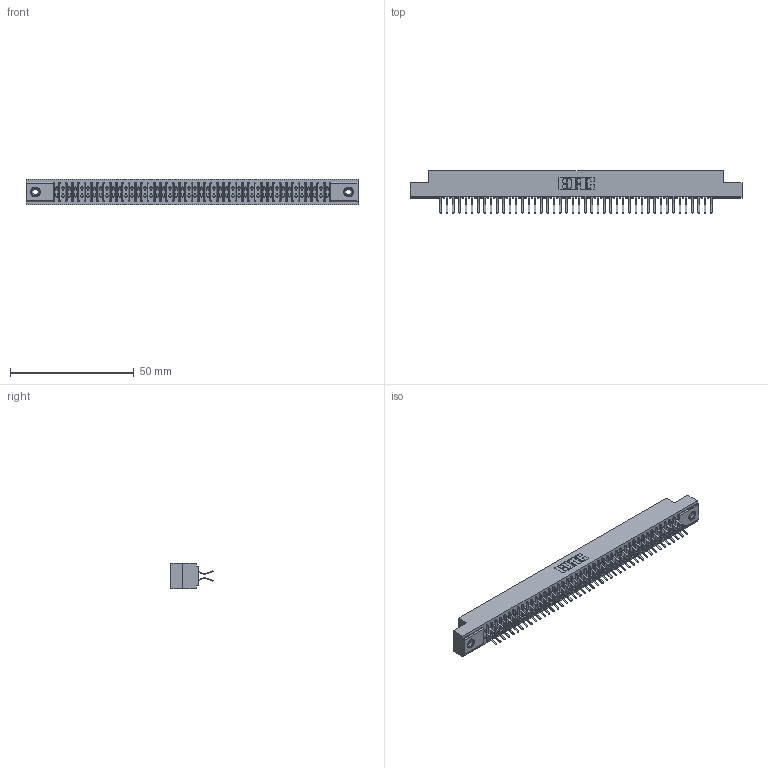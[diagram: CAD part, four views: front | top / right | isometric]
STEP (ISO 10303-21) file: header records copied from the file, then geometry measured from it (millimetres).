
FILE_DESCRIPTION (( 'STEP AP203' ), '1' );
FILE_NAME ('341-088-556-208.STEP', '2018-08-07T23:48:28', ( '' ), ( '' ), 'SwSTEP 2.0', 'SolidWorks 2016', '' );
FILE_SCHEMA (( 'CONFIG_CONTROL_DESIGN' ));
Length unit declared in the file: inch
Products named in the file (4): 341 Part_.156 (3.96) Dia Mounting Holes; 341-292-001_341-292-156; 345-250-001_345-250-003-102; 341-088-556-208
Assembly tree (91 placements, depth 2):
  341-088-556-208
    341 Part_.156 (3.96) Dia Mounting Holes
    341-292-001_341-292-156  x88
    345-250-001_345-250-003-102  x2
Bounding box: 133.99 x 17.07 x 10.16 mm (x, y, z)
Volume: 9917.4 mm3; surface area: 17896.9 mm2
Topology: 91 solids, 91 shells, 6336 faces, 18360 edges, 11906 vertices
Faces by surface type: plane 3620, cylinder 2524, sphere 90, torus 90, cone 12
Entity records: 54308 total; most frequent: CARTESIAN_POINT 9011, ORIENTED_EDGE 8948, DIRECTION 8758, EDGE_CURVE 4474, LINE 3608, VECTOR 3608, VERTEX_POINT 2828, AXIS2_PLACEMENT_3D 2575
